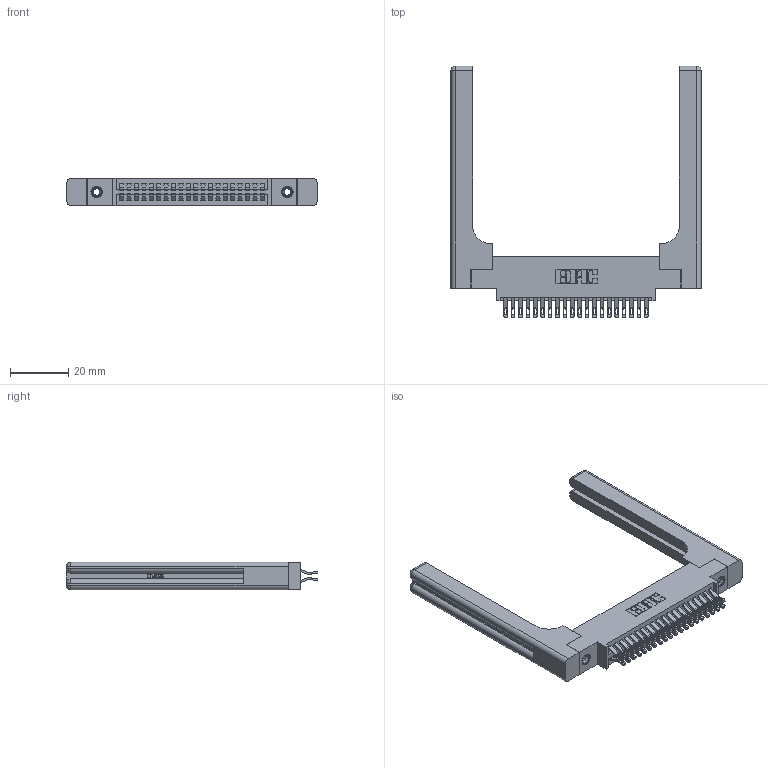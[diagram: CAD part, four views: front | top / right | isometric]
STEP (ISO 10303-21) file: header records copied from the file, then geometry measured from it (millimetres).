
FILE_DESCRIPTION (( 'STEP AP203' ), '1' );
FILE_NAME ('395-040-555-858.STEP', '2019-10-18T05:53:11', ( '' ), ( '' ), 'SwSTEP 2.0', 'SolidWorks 2016', '' );
FILE_SCHEMA (( 'CONFIG_CONTROL_DESIGN' ));
Length unit declared in the file: inch
Products named in the file (5): 345 Part_0.170 Offset - 0.156 Dia-TH; 345-292-001_555 Tail; 345-250-001_345-250-001-102; 345-220-058_345-220-058; 395-040-555-858
Assembly tree (45 placements, depth 2):
  395-040-555-858
    345 Part_0.170 Offset - 0.156 Dia-TH
    345-292-001_555 Tail  x40
    345-250-001_345-250-001-102  x2
    345-220-058_345-220-058  x2
Bounding box: 85.83 x 86.41 x 9.4 mm (x, y, z)
Volume: 16610.8 mm3; surface area: 17205.7 mm2
Topology: 45 solids, 45 shells, 2626 faces, 8099 edges, 5378 vertices
Faces by surface type: plane 1472, cylinder 1094, bspline 36, cone 12, sphere 8, torus 4
Entity records: 24294 total; most frequent: CARTESIAN_POINT 5123, ORIENTED_EDGE 3824, DIRECTION 3444, EDGE_CURVE 1912, VECTOR 1588, LINE 1588, VERTEX_POINT 1266, AXIS2_PLACEMENT_3D 928
